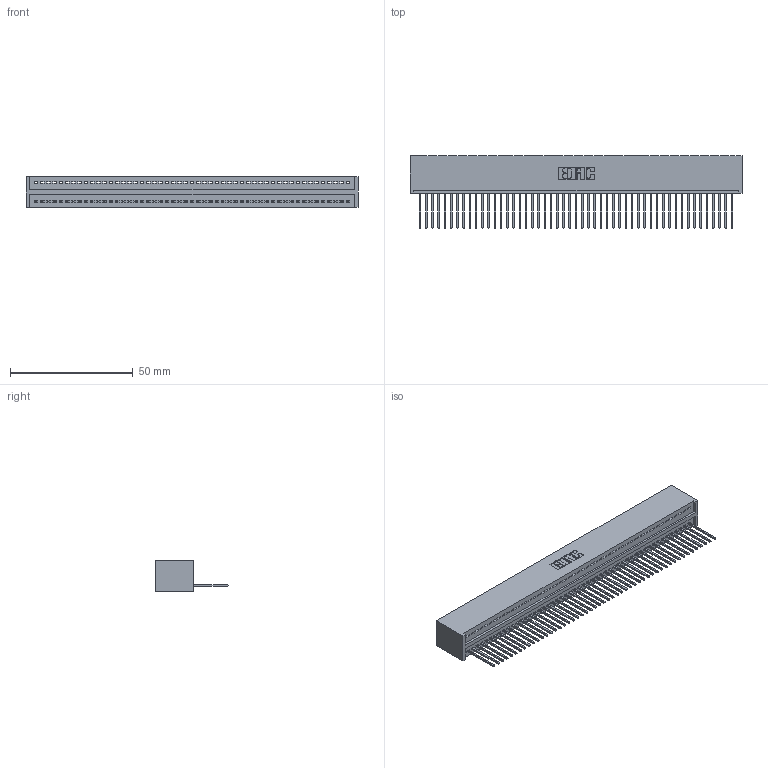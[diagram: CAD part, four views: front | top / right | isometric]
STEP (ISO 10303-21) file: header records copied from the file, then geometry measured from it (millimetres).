
FILE_DESCRIPTION (( 'STEP AP203' ), '1' );
FILE_NAME ('325-051-540-101.STEP', '2020-02-25T00:11:10', ( '' ), ( '' ), 'SwSTEP 2.0', 'SolidWorks 2016', '' );
FILE_SCHEMA (( 'CONFIG_CONTROL_DESIGN' ));
Length unit declared in the file: inch
Products named in the file (3): 325 Part_Lugless; 325-292-001_325-293-140; 325-051-540-101
Assembly tree (52 placements, depth 2):
  325-051-540-101
    325 Part_Lugless
    325-292-001_325-293-140  x51
Bounding box: 135.18 x 29.46 x 12.45 mm (x, y, z)
Volume: 17872.7 mm3; surface area: 20679.8 mm2
Topology: 52 solids, 52 shells, 3064 faces, 9263 edges, 6106 vertices
Faces by surface type: plane 2208, cylinder 856
Entity records: 29755 total; most frequent: CARTESIAN_POINT 5139, ORIENTED_EDGE 5126, DIRECTION 4309, EDGE_CURVE 2563, LINE 2443, VECTOR 2443, VERTEX_POINT 1706, AXIS2_PLACEMENT_3D 933
